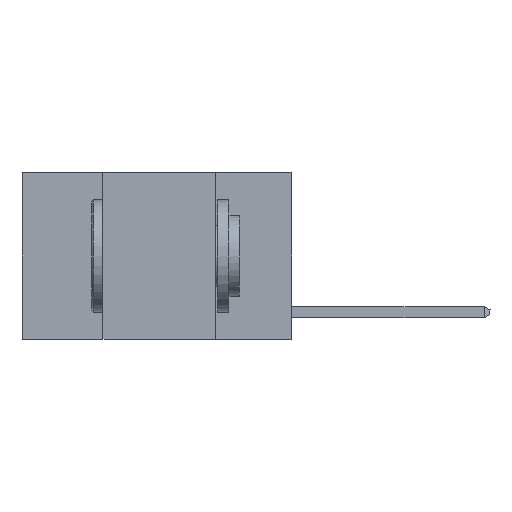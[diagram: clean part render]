
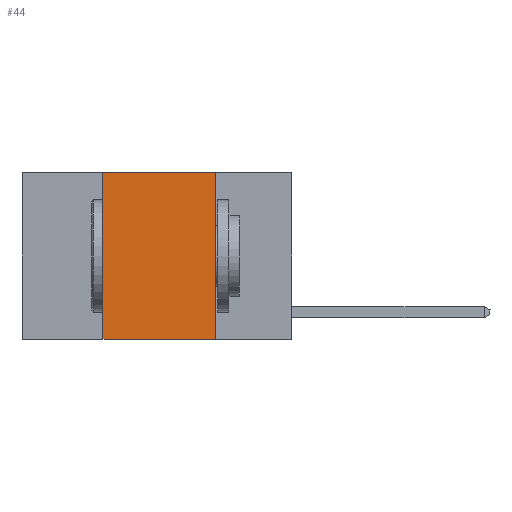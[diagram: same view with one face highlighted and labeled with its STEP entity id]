
A CAD part, left-side view. The second image highlights one B-rep face of the part: STEP entity #44.
In plain terms, the highlighted planar face has unit normal (-1, 0, 0).
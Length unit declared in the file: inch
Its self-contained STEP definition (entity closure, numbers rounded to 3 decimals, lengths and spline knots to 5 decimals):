
#44 = ADVANCED_FACE ( 'NONE', ( #8728 ), #11938, .F. ) ;
#881 = VECTOR ( 'NONE', #9449, 39.37008 ) ;
#1546 = VERTEX_POINT ( 'NONE', #7114 ) ;
#3114 = LINE ( 'NONE', #4583, #881 ) ;
#3180 = EDGE_LOOP ( 'NONE', ( #13909, #7704, #17386, #13365 ) ) ;
#4580 = CARTESIAN_POINT ( 'NONE',  ( 0., 0.42, 0. ) ) ;
#4583 = CARTESIAN_POINT ( 'NONE',  ( 0., 0.6, 0. ) ) ;
#4736 = EDGE_CURVE ( 'NONE', #1546, #20237, #3114, .T. ) ;
#5749 = VECTOR ( 'NONE', #9902, 39.37008 ) ;
#7050 = CARTESIAN_POINT ( 'NONE',  ( 0., 0.17, 0. ) ) ;
#7114 = CARTESIAN_POINT ( 'NONE',  ( 0., 0.42, 0. ) ) ;
#7704 = ORIENTED_EDGE ( 'NONE', *, *, #4736, .F. ) ;
#7754 = VERTEX_POINT ( 'NONE', #9736 ) ;
#8265 = CARTESIAN_POINT ( 'NONE',  ( 0., 0.6, -0.37 ) ) ;
#8453 = VERTEX_POINT ( 'NONE', #15993 ) ;
#8629 = DIRECTION ( 'NONE',  ( 1., 0., 0. ) ) ;
#8728 = FACE_OUTER_BOUND ( 'NONE', #3180, .T. ) ;
#8822 = EDGE_CURVE ( 'NONE', #8453, #1546, #12640, .T. ) ;
#9449 = DIRECTION ( 'NONE',  ( 0., -1., 0. ) ) ;
#9736 = CARTESIAN_POINT ( 'NONE',  ( 0., 0.17, -0.37 ) ) ;
#9902 = DIRECTION ( 'NONE',  ( 0., -1., 0. ) ) ;
#11003 = DIRECTION ( 'NONE',  ( 0., 0., 1. ) ) ;
#11630 = DIRECTION ( 'NONE',  ( 0., 0., -1. ) ) ;
#11938 = PLANE ( 'NONE',  #13707 ) ;
#12640 = LINE ( 'NONE', #4580, #13931 ) ;
#12793 = CARTESIAN_POINT ( 'NONE',  ( 0., 0.6, 0. ) ) ;
#12929 = LINE ( 'NONE', #7050, #17715 ) ;
#13354 = EDGE_CURVE ( 'NONE', #8453, #7754, #17590, .T. ) ;
#13365 = ORIENTED_EDGE ( 'NONE', *, *, #13354, .T. ) ;
#13707 = AXIS2_PLACEMENT_3D ( 'NONE', #12793, #8629, #11630 ) ;
#13909 = ORIENTED_EDGE ( 'NONE', *, *, #14869, .F. ) ;
#13931 = VECTOR ( 'NONE', #11003, 39.37008 ) ;
#14592 = DIRECTION ( 'NONE',  ( 0., 0., -1. ) ) ;
#14869 = EDGE_CURVE ( 'NONE', #20237, #7754, #12929, .T. ) ;
#15000 = CARTESIAN_POINT ( 'NONE',  ( 0., 0.17, 0. ) ) ;
#15993 = CARTESIAN_POINT ( 'NONE',  ( 0., 0.42, -0.37 ) ) ;
#17386 = ORIENTED_EDGE ( 'NONE', *, *, #8822, .F. ) ;
#17590 = LINE ( 'NONE', #8265, #5749 ) ;
#17715 = VECTOR ( 'NONE', #14592, 39.37008 ) ;
#20237 = VERTEX_POINT ( 'NONE', #15000 ) ;
